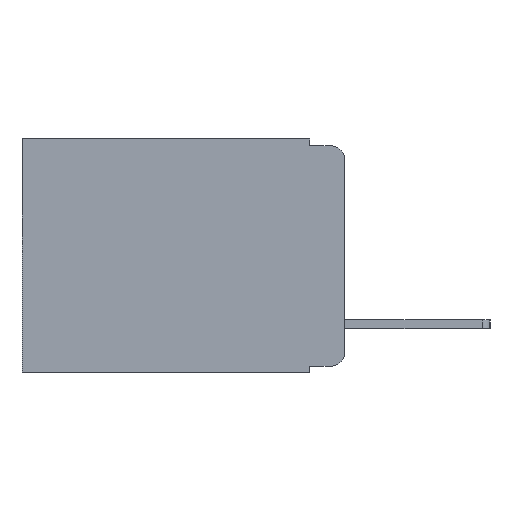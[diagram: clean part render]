
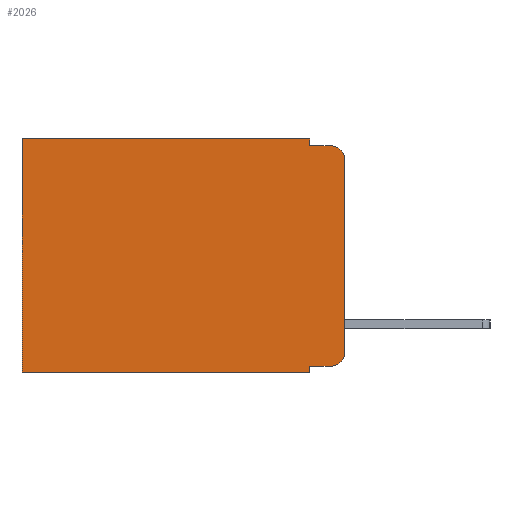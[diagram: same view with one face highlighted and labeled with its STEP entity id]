
A CAD part, left-side view. The second image highlights one B-rep face of the part: STEP entity #2026.
In plain terms, the highlighted planar face has unit normal (-1, 0, 0).
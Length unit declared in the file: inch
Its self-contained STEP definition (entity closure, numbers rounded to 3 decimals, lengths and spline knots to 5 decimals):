
#58 = VERTEX_POINT ( 'NONE', #10971 ) ;
#208 = VERTEX_POINT ( 'NONE', #11484 ) ;
#325 = EDGE_CURVE ( 'NONE', #8765, #757, #11682, .T. ) ;
#451 = AXIS2_PLACEMENT_3D ( 'NONE', #2992, #9275, #4136 ) ;
#699 = VERTEX_POINT ( 'NONE', #7506 ) ;
#757 = VERTEX_POINT ( 'NONE', #941 ) ;
#804 = EDGE_CURVE ( 'NONE', #7579, #208, #11911, .T. ) ;
#915 = DIRECTION ( 'NONE',  ( 0., 0., -1. ) ) ;
#941 = CARTESIAN_POINT ( 'NONE',  ( 0.298, 0.473, -0.343 ) ) ;
#1229 = EDGE_CURVE ( 'NONE', #4422, #7579, #5776, .T. ) ;
#1507 = DIRECTION ( 'NONE',  ( 0., 0., -1. ) ) ;
#1612 = VECTOR ( 'NONE', #7874, 39.37008 ) ;
#1733 = VERTEX_POINT ( 'NONE', #4216 ) ;
#1798 = LINE ( 'NONE', #11062, #11197 ) ;
#1846 = EDGE_CURVE ( 'NONE', #58, #208, #4397, .T. ) ;
#1863 = PLANE ( 'NONE',  #3320 ) ;
#1927 = CARTESIAN_POINT ( 'NONE',  ( 0.298, 0.051, -0.01 ) ) ;
#2026 = ADVANCED_FACE ( 'NONE', ( #7249 ), #1863, .F. ) ;
#2093 = CARTESIAN_POINT ( 'NONE',  ( 0.298, 0.051, -0.01 ) ) ;
#2334 = LINE ( 'NONE', #2651, #11325 ) ;
#2485 = VERTEX_POINT ( 'NONE', #5707 ) ;
#2540 = AXIS2_PLACEMENT_3D ( 'NONE', #10131, #11186, #5332 ) ;
#2651 = CARTESIAN_POINT ( 'NONE',  ( 0.298, 0.473, 0. ) ) ;
#2992 = CARTESIAN_POINT ( 'NONE',  ( 0.298, 0.02, -0.313 ) ) ;
#3090 = ORIENTED_EDGE ( 'NONE', *, *, #5778, .T. ) ;
#3263 = DIRECTION ( 'NONE',  ( 0., 1., 0. ) ) ;
#3320 = AXIS2_PLACEMENT_3D ( 'NONE', #6594, #11403, #11381 ) ;
#3727 = CIRCLE ( 'NONE', #451, 0.02 ) ;
#3741 = LINE ( 'NONE', #5124, #10388 ) ;
#4073 = DIRECTION ( 'NONE',  ( 0., -1., 0. ) ) ;
#4136 = DIRECTION ( 'NONE',  ( 0., 0., -1. ) ) ;
#4143 = ORIENTED_EDGE ( 'NONE', *, *, #5275, .T. ) ;
#4216 = CARTESIAN_POINT ( 'NONE',  ( 0.298, 0., -0.313 ) ) ;
#4397 = CIRCLE ( 'NONE', #2540, 0.02 ) ;
#4407 = ORIENTED_EDGE ( 'NONE', *, *, #4563, .T. ) ;
#4422 = VERTEX_POINT ( 'NONE', #10190 ) ;
#4547 = CARTESIAN_POINT ( 'NONE',  ( 0.298, 0.051, -0.343 ) ) ;
#4563 = EDGE_CURVE ( 'NONE', #4422, #5802, #10140, .T. ) ;
#4564 = ORIENTED_EDGE ( 'NONE', *, *, #7385, .T. ) ;
#5080 = ORIENTED_EDGE ( 'NONE', *, *, #5134, .F. ) ;
#5124 = CARTESIAN_POINT ( 'NONE',  ( 0.298, 0.051, 0. ) ) ;
#5134 = EDGE_CURVE ( 'NONE', #58, #1733, #1798, .T. ) ;
#5165 = EDGE_CURVE ( 'NONE', #699, #8765, #3741, .T. ) ;
#5275 = EDGE_CURVE ( 'NONE', #699, #2485, #9069, .T. ) ;
#5332 = DIRECTION ( 'NONE',  ( 0., 0., -1. ) ) ;
#5707 = CARTESIAN_POINT ( 'NONE',  ( 0.298, 0.02, -0.333 ) ) ;
#5776 = LINE ( 'NONE', #6777, #8049 ) ;
#5778 = EDGE_CURVE ( 'NONE', #5802, #757, #2334, .T. ) ;
#5802 = VERTEX_POINT ( 'NONE', #9837 ) ;
#5981 = CARTESIAN_POINT ( 'NONE',  ( 0.298, 0., -0.343 ) ) ;
#6169 = CARTESIAN_POINT ( 'NONE',  ( 0.298, 0.051, -0.333 ) ) ;
#6183 = ORIENTED_EDGE ( 'NONE', *, *, #1229, .F. ) ;
#6594 = CARTESIAN_POINT ( 'NONE',  ( 0.298, 0., 0. ) ) ;
#6777 = CARTESIAN_POINT ( 'NONE',  ( 0.298, 0.051, 0. ) ) ;
#7249 = FACE_OUTER_BOUND ( 'NONE', #9241, .T. ) ;
#7385 = EDGE_CURVE ( 'NONE', #2485, #1733, #3727, .T. ) ;
#7506 = CARTESIAN_POINT ( 'NONE',  ( 0.298, 0.051, -0.333 ) ) ;
#7579 = VERTEX_POINT ( 'NONE', #2093 ) ;
#7874 = DIRECTION ( 'NONE',  ( 0., -1., 0. ) ) ;
#7903 = VECTOR ( 'NONE', #9525, 39.37008 ) ;
#8049 = VECTOR ( 'NONE', #10300, 39.37008 ) ;
#8165 = ORIENTED_EDGE ( 'NONE', *, *, #1846, .T. ) ;
#8657 = CARTESIAN_POINT ( 'NONE',  ( 0.298, 0., 0. ) ) ;
#8765 = VERTEX_POINT ( 'NONE', #4547 ) ;
#8836 = ORIENTED_EDGE ( 'NONE', *, *, #804, .F. ) ;
#8976 = ORIENTED_EDGE ( 'NONE', *, *, #5165, .F. ) ;
#9069 = LINE ( 'NONE', #6169, #1612 ) ;
#9241 = EDGE_LOOP ( 'NONE', ( #5080, #8165, #8836, #6183, #4407, #3090, #11460, #8976, #4143, #4564 ) ) ;
#9275 = DIRECTION ( 'NONE',  ( -1., 0., 0. ) ) ;
#9525 = DIRECTION ( 'NONE',  ( 0., 1., 0. ) ) ;
#9837 = CARTESIAN_POINT ( 'NONE',  ( 0.298, 0.473, 0. ) ) ;
#10131 = CARTESIAN_POINT ( 'NONE',  ( 0.298, 0.02, -0.03 ) ) ;
#10140 = LINE ( 'NONE', #8657, #7903 ) ;
#10190 = CARTESIAN_POINT ( 'NONE',  ( 0.298, 0.051, 0. ) ) ;
#10300 = DIRECTION ( 'NONE',  ( 0., 0., -1. ) ) ;
#10388 = VECTOR ( 'NONE', #915, 39.37008 ) ;
#10971 = CARTESIAN_POINT ( 'NONE',  ( 0.298, 0., -0.03 ) ) ;
#11062 = CARTESIAN_POINT ( 'NONE',  ( 0.298, 0., 0. ) ) ;
#11186 = DIRECTION ( 'NONE',  ( -1., 0., 0. ) ) ;
#11197 = VECTOR ( 'NONE', #11845, 39.37008 ) ;
#11325 = VECTOR ( 'NONE', #1507, 39.37008 ) ;
#11381 = DIRECTION ( 'NONE',  ( 0., 0., -1. ) ) ;
#11403 = DIRECTION ( 'NONE',  ( 1., 0., 0. ) ) ;
#11452 = VECTOR ( 'NONE', #3263, 39.37008 ) ;
#11460 = ORIENTED_EDGE ( 'NONE', *, *, #325, .F. ) ;
#11484 = CARTESIAN_POINT ( 'NONE',  ( 0.298, 0.02, -0.01 ) ) ;
#11660 = VECTOR ( 'NONE', #4073, 39.37008 ) ;
#11682 = LINE ( 'NONE', #5981, #11452 ) ;
#11845 = DIRECTION ( 'NONE',  ( 0., 0., -1. ) ) ;
#11911 = LINE ( 'NONE', #1927, #11660 ) ;
